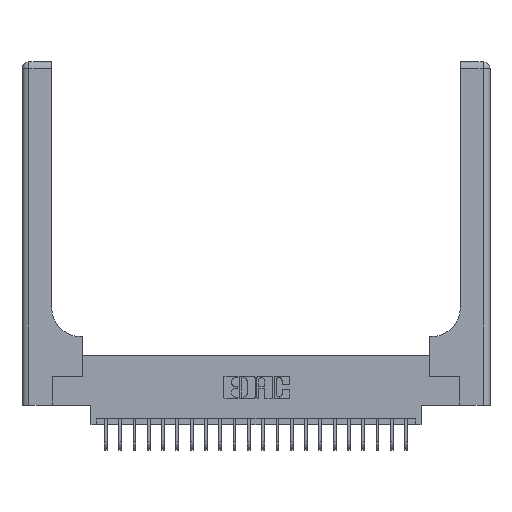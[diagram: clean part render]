
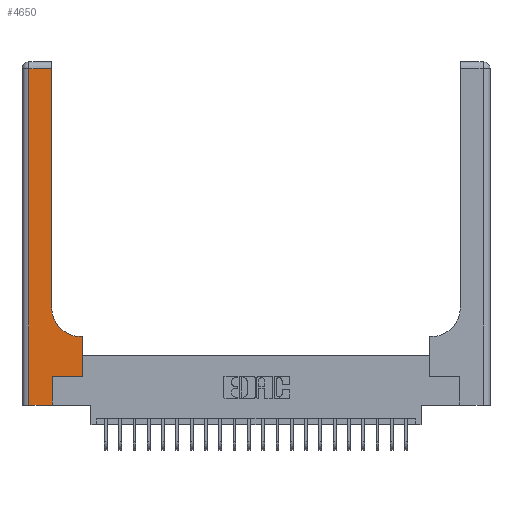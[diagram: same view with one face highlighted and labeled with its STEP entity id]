
A CAD part, top view. The second image highlights one B-rep face of the part: STEP entity #4650.
In plain terms, the highlighted planar face has unit normal (0, 0, 1).
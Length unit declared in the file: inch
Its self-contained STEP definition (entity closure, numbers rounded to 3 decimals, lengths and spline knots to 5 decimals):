
#58 = EDGE_CURVE ( 'NONE', #21802, #12846, #17123, .T. ) ;
#163 = DIRECTION ( 'NONE',  ( 0., 1., 0. ) ) ;
#264 = DIRECTION ( 'NONE',  ( 1., 0., 0. ) ) ;
#433 = ORIENTED_EDGE ( 'NONE', *, *, #1292, .T. ) ;
#690 = ORIENTED_EDGE ( 'NONE', *, *, #22636, .T. ) ;
#825 = ORIENTED_EDGE ( 'NONE', *, *, #7880, .T. ) ;
#896 = CARTESIAN_POINT ( 'NONE',  ( 0.26, 0.85, 0.37 ) ) ;
#1089 = CARTESIAN_POINT ( 'NONE',  ( 0.528, 0.25, 0.37 ) ) ;
#1292 = EDGE_CURVE ( 'NONE', #12445, #21802, #17340, .T. ) ;
#1809 = CARTESIAN_POINT ( 'NONE',  ( 0.265, 0.25, 0.37 ) ) ;
#2792 = AXIS2_PLACEMENT_3D ( 'NONE', #13214, #15199, #9345 ) ;
#3316 = VERTEX_POINT ( 'NONE', #22891 ) ;
#3537 = CARTESIAN_POINT ( 'NONE',  ( 0.51, 0.6, 0.37 ) ) ;
#3704 = LINE ( 'NONE', #22639, #10803 ) ;
#3922 = DIRECTION ( 'NONE',  ( 1., 0., 0. ) ) ;
#4232 = DIRECTION ( 'NONE',  ( 0., 0., -1. ) ) ;
#4650 = ADVANCED_FACE ( 'NONE', ( #9725 ), #22428, .F. ) ;
#5026 = EDGE_CURVE ( 'NONE', #11188, #12445, #11028, .T. ) ;
#5417 = CARTESIAN_POINT ( 'NONE',  ( 0., 0., 0.37 ) ) ;
#5783 = ORIENTED_EDGE ( 'NONE', *, *, #16944, .T. ) ;
#7159 = LINE ( 'NONE', #1089, #8075 ) ;
#7575 = AXIS2_PLACEMENT_3D ( 'NONE', #17680, #4232, #264 ) ;
#7578 = ORIENTED_EDGE ( 'NONE', *, *, #18474, .T. ) ;
#7761 = CARTESIAN_POINT ( 'NONE',  ( 0.265, 0., 0.37 ) ) ;
#7880 = EDGE_CURVE ( 'NONE', #12846, #19666, #7159, .T. ) ;
#8075 = VECTOR ( 'NONE', #14764, 39.37008 ) ;
#8247 = LINE ( 'NONE', #17714, #19568 ) ;
#8623 = VERTEX_POINT ( 'NONE', #3537 ) ;
#9345 = DIRECTION ( 'NONE',  ( -1., 0., 0. ) ) ;
#9725 = FACE_OUTER_BOUND ( 'NONE', #17071, .T. ) ;
#9888 = VECTOR ( 'NONE', #163, 39.37008 ) ;
#10227 = ORIENTED_EDGE ( 'NONE', *, *, #5026, .T. ) ;
#10615 = CARTESIAN_POINT ( 'NONE',  ( 0.265, 0.25, 0.37 ) ) ;
#10652 = DIRECTION ( 'NONE',  ( 1., 0., 0. ) ) ;
#10803 = VECTOR ( 'NONE', #18527, 39.37008 ) ;
#10987 = LINE ( 'NONE', #24437, #17264 ) ;
#11028 = LINE ( 'NONE', #5417, #15544 ) ;
#11188 = VERTEX_POINT ( 'NONE', #17350 ) ;
#11852 = CARTESIAN_POINT ( 'NONE',  ( 0.265, 0., 0.37 ) ) ;
#12445 = VERTEX_POINT ( 'NONE', #7761 ) ;
#12761 = DIRECTION ( 'NONE',  ( 0., 1., 0. ) ) ;
#12846 = VERTEX_POINT ( 'NONE', #18136 ) ;
#12894 = CARTESIAN_POINT ( 'NONE',  ( 0.26, 3., 0.37 ) ) ;
#13214 = CARTESIAN_POINT ( 'NONE',  ( 0., 3., 0.37 ) ) ;
#13691 = VECTOR ( 'NONE', #12761, 39.37008 ) ;
#14507 = LINE ( 'NONE', #12894, #13691 ) ;
#14764 = DIRECTION ( 'NONE',  ( 0., 1., 0. ) ) ;
#15199 = DIRECTION ( 'NONE',  ( 0., 0., -1. ) ) ;
#15368 = ORIENTED_EDGE ( 'NONE', *, *, #19683, .T. ) ;
#15544 = VECTOR ( 'NONE', #10652, 39.37008 ) ;
#16203 = DIRECTION ( 'NONE',  ( -1., 0., 0. ) ) ;
#16826 = ORIENTED_EDGE ( 'NONE', *, *, #22006, .T. ) ;
#16944 = EDGE_CURVE ( 'NONE', #8623, #19698, #23880, .T. ) ;
#17071 = EDGE_LOOP ( 'NONE', ( #690, #16826, #7578, #10227, #433, #20549, #825, #15368, #5783 ) ) ;
#17123 = LINE ( 'NONE', #1809, #20386 ) ;
#17264 = VECTOR ( 'NONE', #18582, 39.37008 ) ;
#17340 = LINE ( 'NONE', #11852, #9888 ) ;
#17350 = CARTESIAN_POINT ( 'NONE',  ( 0.06, 0., 0.37 ) ) ;
#17680 = CARTESIAN_POINT ( 'NONE',  ( 0.51, 0.85, 0.37 ) ) ;
#17714 = CARTESIAN_POINT ( 'NONE',  ( 0.26, 0.6, 0.37 ) ) ;
#17950 = CARTESIAN_POINT ( 'NONE',  ( 0.528, 0.6, 0.37 ) ) ;
#18004 = CARTESIAN_POINT ( 'NONE',  ( 0.06, 2.94, 0.37 ) ) ;
#18136 = CARTESIAN_POINT ( 'NONE',  ( 0.528, 0.25, 0.37 ) ) ;
#18474 = EDGE_CURVE ( 'NONE', #22584, #11188, #3704, .T. ) ;
#18527 = DIRECTION ( 'NONE',  ( 0., -1., 0. ) ) ;
#18582 = DIRECTION ( 'NONE',  ( -1., 0., 0. ) ) ;
#19568 = VECTOR ( 'NONE', #16203, 39.37008 ) ;
#19666 = VERTEX_POINT ( 'NONE', #17950 ) ;
#19683 = EDGE_CURVE ( 'NONE', #19666, #8623, #8247, .T. ) ;
#19698 = VERTEX_POINT ( 'NONE', #896 ) ;
#20386 = VECTOR ( 'NONE', #3922, 39.37008 ) ;
#20549 = ORIENTED_EDGE ( 'NONE', *, *, #58, .T. ) ;
#21802 = VERTEX_POINT ( 'NONE', #10615 ) ;
#22006 = EDGE_CURVE ( 'NONE', #3316, #22584, #10987, .T. ) ;
#22428 = PLANE ( 'NONE',  #2792 ) ;
#22584 = VERTEX_POINT ( 'NONE', #18004 ) ;
#22636 = EDGE_CURVE ( 'NONE', #19698, #3316, #14507, .T. ) ;
#22639 = CARTESIAN_POINT ( 'NONE',  ( 0.06, 3., 0.37 ) ) ;
#22891 = CARTESIAN_POINT ( 'NONE',  ( 0.26, 2.94, 0.37 ) ) ;
#23880 = CIRCLE ( 'NONE', #7575, 0.25 ) ;
#24437 = CARTESIAN_POINT ( 'NONE',  ( 0., 2.94, 0.37 ) ) ;
